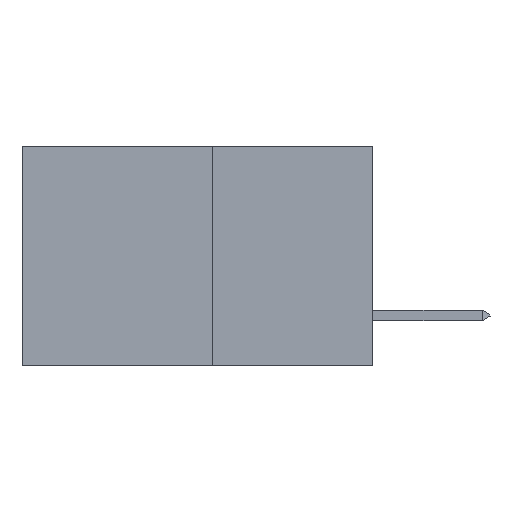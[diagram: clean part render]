
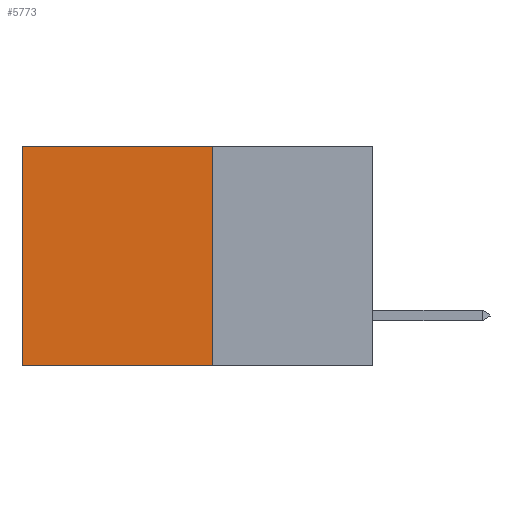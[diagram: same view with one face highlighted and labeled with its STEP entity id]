
A CAD part, left-side view. The second image highlights one B-rep face of the part: STEP entity #5773.
In plain terms, the highlighted planar face has unit normal (-1, 0, 0).
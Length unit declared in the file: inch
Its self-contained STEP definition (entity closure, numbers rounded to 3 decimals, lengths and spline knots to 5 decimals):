
#1212 = PLANE ( 'NONE',  #12560 ) ;
#1440 = VECTOR ( 'NONE', #2803, 39.37008 ) ;
#1551 = EDGE_CURVE ( 'NONE', #2755, #6195, #3957, .T. ) ;
#1570 = VERTEX_POINT ( 'NONE', #4361 ) ;
#1689 = DIRECTION ( 'NONE',  ( 0., 0., -1. ) ) ;
#2148 = EDGE_CURVE ( 'NONE', #2755, #12608, #5467, .T. ) ;
#2174 = EDGE_CURVE ( 'NONE', #12608, #1570, #14250, .T. ) ;
#2421 = DIRECTION ( 'NONE',  ( 0., 0., -1. ) ) ;
#2755 = VERTEX_POINT ( 'NONE', #13399 ) ;
#2803 = DIRECTION ( 'NONE',  ( 0., 1., 0. ) ) ;
#2958 = CARTESIAN_POINT ( 'NONE',  ( 0.277, 0.27, -0.37 ) ) ;
#2983 = VECTOR ( 'NONE', #10381, 39.37008 ) ;
#3561 = VECTOR ( 'NONE', #12809, 39.37008 ) ;
#3957 = LINE ( 'NONE', #11883, #3561 ) ;
#4361 = CARTESIAN_POINT ( 'NONE',  ( 0.277, 0.59, -0.37 ) ) ;
#5467 = LINE ( 'NONE', #5784, #11081 ) ;
#5679 = ORIENTED_EDGE ( 'NONE', *, *, #1551, .T. ) ;
#5773 = ADVANCED_FACE ( 'NONE', ( #5787 ), #1212, .F. ) ;
#5784 = CARTESIAN_POINT ( 'NONE',  ( 0.277, 0.27, -0.37 ) ) ;
#5787 = FACE_OUTER_BOUND ( 'NONE', #11185, .T. ) ;
#6195 = VERTEX_POINT ( 'NONE', #8867 ) ;
#6619 = ORIENTED_EDGE ( 'NONE', *, *, #10462, .T. ) ;
#7145 = CARTESIAN_POINT ( 'NONE',  ( 0.277, 0.27, -0.37 ) ) ;
#7750 = ORIENTED_EDGE ( 'NONE', *, *, #2174, .F. ) ;
#8431 = CARTESIAN_POINT ( 'NONE',  ( 0.277, 0.27, -0.37 ) ) ;
#8867 = CARTESIAN_POINT ( 'NONE',  ( 0.277, 0.59, 0. ) ) ;
#9195 = CARTESIAN_POINT ( 'NONE',  ( 0.277, 0.59, -0.37 ) ) ;
#9683 = DIRECTION ( 'NONE',  ( 1., 0., 0. ) ) ;
#10381 = DIRECTION ( 'NONE',  ( 0., 0., -1. ) ) ;
#10462 = EDGE_CURVE ( 'NONE', #6195, #1570, #12597, .T. ) ;
#11081 = VECTOR ( 'NONE', #1689, 39.37008 ) ;
#11185 = EDGE_LOOP ( 'NONE', ( #6619, #7750, #11279, #5679 ) ) ;
#11279 = ORIENTED_EDGE ( 'NONE', *, *, #2148, .F. ) ;
#11883 = CARTESIAN_POINT ( 'NONE',  ( 0.277, 0.27, 0. ) ) ;
#12560 = AXIS2_PLACEMENT_3D ( 'NONE', #8431, #9683, #2421 ) ;
#12597 = LINE ( 'NONE', #9195, #2983 ) ;
#12608 = VERTEX_POINT ( 'NONE', #7145 ) ;
#12809 = DIRECTION ( 'NONE',  ( 0., 1., 0. ) ) ;
#13399 = CARTESIAN_POINT ( 'NONE',  ( 0.277, 0.27, 0. ) ) ;
#14250 = LINE ( 'NONE', #2958, #1440 ) ;
